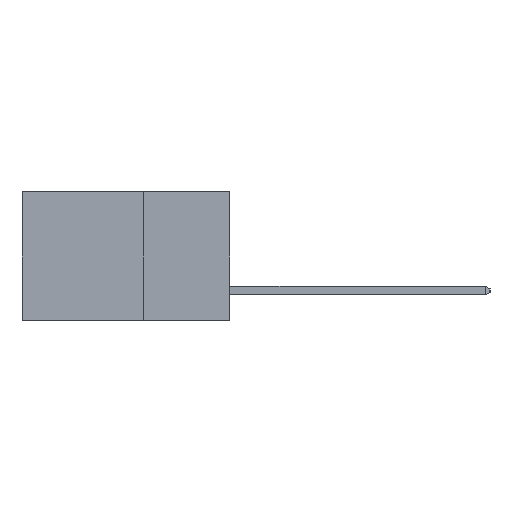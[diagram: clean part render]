
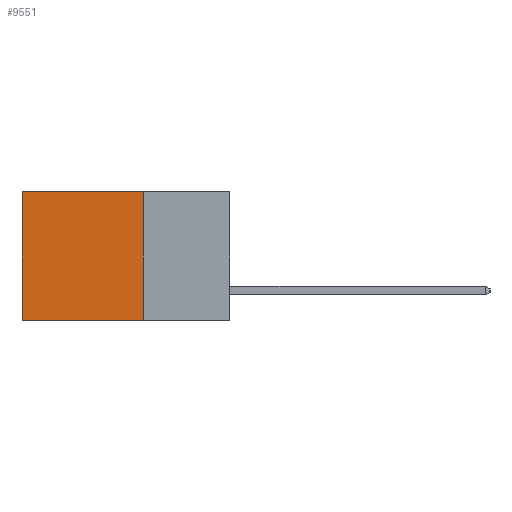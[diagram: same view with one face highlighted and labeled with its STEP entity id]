
A CAD part, left-side view. The second image highlights one B-rep face of the part: STEP entity #9551.
In plain terms, the highlighted planar face has unit normal (-1, 0, 0).
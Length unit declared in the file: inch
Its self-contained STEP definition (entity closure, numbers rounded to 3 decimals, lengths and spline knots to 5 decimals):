
#318 = VERTEX_POINT ( 'NONE', #7771 ) ;
#1038 = VERTEX_POINT ( 'NONE', #10722 ) ;
#1051 = EDGE_CURVE ( 'NONE', #1038, #16404, #8719, .T. ) ;
#2696 = EDGE_CURVE ( 'NONE', #8340, #16404, #19107, .T. ) ;
#3268 = VECTOR ( 'NONE', #9277, 39.37008 ) ;
#5711 = ORIENTED_EDGE ( 'NONE', *, *, #2696, .F. ) ;
#6007 = DIRECTION ( 'NONE',  ( 0., 1., 0. ) ) ;
#6190 = CARTESIAN_POINT ( 'NONE',  ( 0.2615, 0.25, 0. ) ) ;
#7771 = CARTESIAN_POINT ( 'NONE',  ( 0.2615, 0.25, 0. ) ) ;
#8042 = CARTESIAN_POINT ( 'NONE',  ( 0.2615, 0.25, -0.37 ) ) ;
#8340 = VERTEX_POINT ( 'NONE', #17020 ) ;
#8390 = CARTESIAN_POINT ( 'NONE',  ( 0.2615, 0.6, -0.37 ) ) ;
#8719 = LINE ( 'NONE', #12451, #16881 ) ;
#8757 = EDGE_LOOP ( 'NONE', ( #9939, #5711, #13208, #9647 ) ) ;
#8854 = CARTESIAN_POINT ( 'NONE',  ( 0.2615, 0.25, -0.37 ) ) ;
#9050 = FACE_OUTER_BOUND ( 'NONE', #8757, .T. ) ;
#9277 = DIRECTION ( 'NONE',  ( 0., 1., 0. ) ) ;
#9551 = ADVANCED_FACE ( 'NONE', ( #9050 ), #12079, .F. ) ;
#9613 = DIRECTION ( 'NONE',  ( 0., 0., -1. ) ) ;
#9647 = ORIENTED_EDGE ( 'NONE', *, *, #9855, .T. ) ;
#9855 = EDGE_CURVE ( 'NONE', #318, #1038, #15544, .T. ) ;
#9939 = ORIENTED_EDGE ( 'NONE', *, *, #1051, .T. ) ;
#10474 = VECTOR ( 'NONE', #9613, 39.37008 ) ;
#10722 = CARTESIAN_POINT ( 'NONE',  ( 0.2615, 0.6, 0. ) ) ;
#10956 = LINE ( 'NONE', #8042, #10474 ) ;
#11907 = EDGE_CURVE ( 'NONE', #318, #8340, #10956, .T. ) ;
#12021 = DIRECTION ( 'NONE',  ( 0., 0., -1. ) ) ;
#12030 = DIRECTION ( 'NONE',  ( 1., 0., 0. ) ) ;
#12048 = CARTESIAN_POINT ( 'NONE',  ( 0.2615, 0.25, -0.37 ) ) ;
#12079 = PLANE ( 'NONE',  #13126 ) ;
#12137 = DIRECTION ( 'NONE',  ( 0., 0., -1. ) ) ;
#12451 = CARTESIAN_POINT ( 'NONE',  ( 0.2615, 0.6, -0.37 ) ) ;
#13126 = AXIS2_PLACEMENT_3D ( 'NONE', #12048, #12030, #12021 ) ;
#13208 = ORIENTED_EDGE ( 'NONE', *, *, #11907, .F. ) ;
#15544 = LINE ( 'NONE', #6190, #19890 ) ;
#16404 = VERTEX_POINT ( 'NONE', #8390 ) ;
#16881 = VECTOR ( 'NONE', #12137, 39.37008 ) ;
#17020 = CARTESIAN_POINT ( 'NONE',  ( 0.2615, 0.25, -0.37 ) ) ;
#19107 = LINE ( 'NONE', #8854, #3268 ) ;
#19890 = VECTOR ( 'NONE', #6007, 39.37008 ) ;
